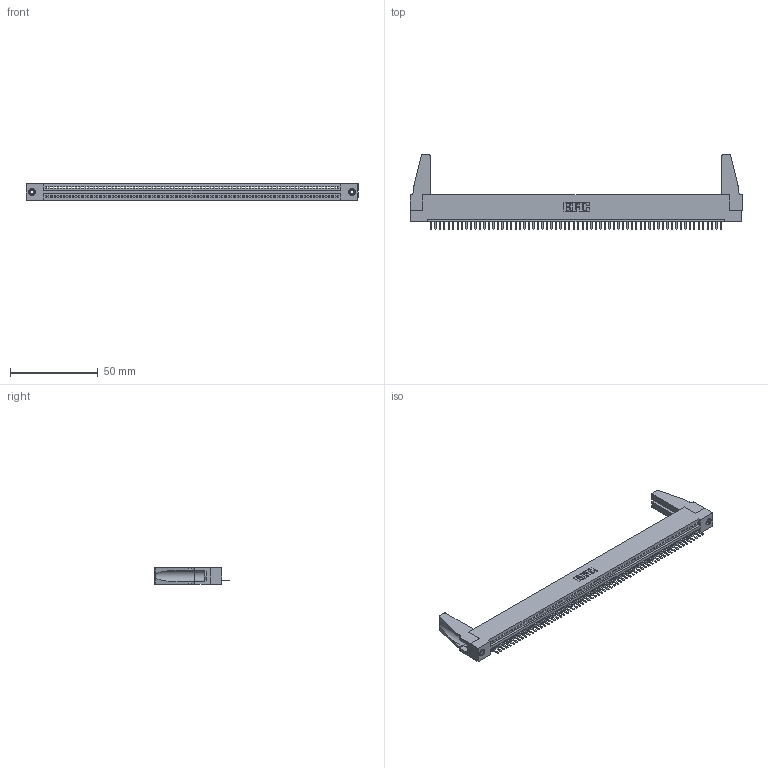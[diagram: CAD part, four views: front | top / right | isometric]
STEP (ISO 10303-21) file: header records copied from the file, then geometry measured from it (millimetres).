
FILE_DESCRIPTION (( 'STEP AP203' ), '1' );
FILE_NAME ('345-066-520-188.STEP', '2019-10-11T20:07:01', ( '' ), ( '' ), 'SwSTEP 2.0', 'SolidWorks 2016', '' );
FILE_SCHEMA (( 'CONFIG_CONTROL_DESIGN' ));
Length unit declared in the file: inch
Products named in the file (5): 345 Part_Flush Mounting Lugs - 0.156 Dia-TH; 345-250-001_345-250-001-102; 345-066-520-188; 345-292-001_345-293-120; 345-220-078_345-220-088
Assembly tree (71 placements, depth 2):
  345-066-520-188
    345 Part_Flush Mounting Lugs - 0.156 Dia-TH
    345-292-001_345-293-120  x66
    345-250-001_345-250-001-102  x2
    345-220-078_345-220-088  x2
Bounding box: 188.87 x 42.55 x 9.4 mm (x, y, z)
Volume: 21198.7 mm3; surface area: 26683.3 mm2
Topology: 71 solids, 71 shells, 4342 faces, 12799 edges, 8346 vertices
Faces by surface type: plane 2924, cylinder 1402, cone 12, torus 4
Entity records: 48704 total; most frequent: CARTESIAN_POINT 8436, ORIENTED_EDGE 8384, DIRECTION 7328, EDGE_CURVE 4192, LINE 3750, VECTOR 3750, VERTEX_POINT 2786, AXIS2_PLACEMENT_3D 1789
